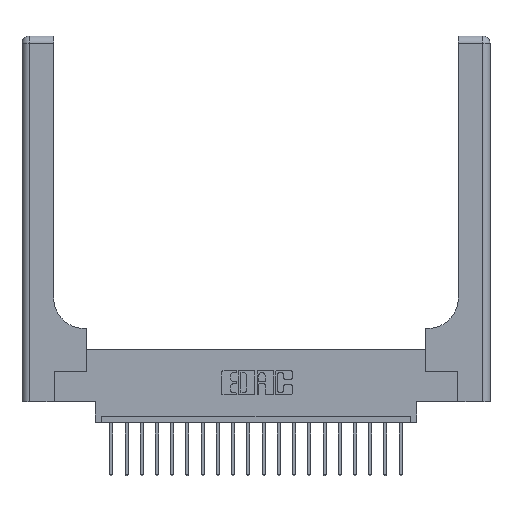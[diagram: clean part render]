
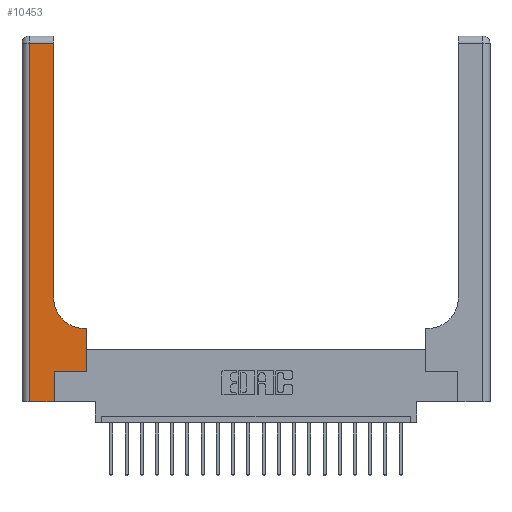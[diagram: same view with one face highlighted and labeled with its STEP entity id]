
A CAD part, top view. The second image highlights one B-rep face of the part: STEP entity #10453.
In plain terms, the highlighted planar face has unit normal (0, 0, 1).
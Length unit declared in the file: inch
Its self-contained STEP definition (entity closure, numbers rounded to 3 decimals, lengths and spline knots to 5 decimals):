
#412 = EDGE_CURVE ( 'NONE', #14794, #13893, #10977, .T. ) ;
#609 = DIRECTION ( 'NONE',  ( 1., 0., 0. ) ) ;
#1323 = VERTEX_POINT ( 'NONE', #8451 ) ;
#1460 = DIRECTION ( 'NONE',  ( 0., 0., -1. ) ) ;
#1505 = CARTESIAN_POINT ( 'NONE',  ( 0.06, 3., 0.37 ) ) ;
#1817 = ORIENTED_EDGE ( 'NONE', *, *, #3419, .T. ) ;
#2154 = ORIENTED_EDGE ( 'NONE', *, *, #20997, .T. ) ;
#2956 = CARTESIAN_POINT ( 'NONE',  ( 0., 3., 0.37 ) ) ;
#2967 = DIRECTION ( 'NONE',  ( 0., 1., 0. ) ) ;
#3419 = EDGE_CURVE ( 'NONE', #13768, #9009, #17662, .T. ) ;
#3520 = VECTOR ( 'NONE', #11251, 39.37008 ) ;
#3638 = VECTOR ( 'NONE', #9636, 39.37008 ) ;
#4428 = AXIS2_PLACEMENT_3D ( 'NONE', #9520, #8522, #15043 ) ;
#4526 = CARTESIAN_POINT ( 'NONE',  ( 0.06, 0., 0.37 ) ) ;
#4761 = VECTOR ( 'NONE', #16484, 39.37008 ) ;
#4892 = CARTESIAN_POINT ( 'NONE',  ( 0.528, 0.6, 0.37 ) ) ;
#5689 = VERTEX_POINT ( 'NONE', #10002 ) ;
#6119 = CARTESIAN_POINT ( 'NONE',  ( 0.26, 3., 0.37 ) ) ;
#6524 = VERTEX_POINT ( 'NONE', #8384 ) ;
#6579 = ORIENTED_EDGE ( 'NONE', *, *, #8821, .T. ) ;
#7042 = EDGE_CURVE ( 'NONE', #13893, #6524, #12755, .T. ) ;
#7211 = EDGE_LOOP ( 'NONE', ( #13120, #1817, #12132, #15295, #9755, #7879, #6579, #2154, #18688 ) ) ;
#7524 = EDGE_CURVE ( 'NONE', #5689, #1323, #10559, .T. ) ;
#7879 = ORIENTED_EDGE ( 'NONE', *, *, #7042, .T. ) ;
#7968 = DIRECTION ( 'NONE',  ( -1., 0., 0. ) ) ;
#8384 = CARTESIAN_POINT ( 'NONE',  ( 0.528, 0.25, 0.37 ) ) ;
#8451 = CARTESIAN_POINT ( 'NONE',  ( 0.26, 0.85, 0.37 ) ) ;
#8522 = DIRECTION ( 'NONE',  ( 0., 0., -1. ) ) ;
#8564 = LINE ( 'NONE', #18298, #4761 ) ;
#8821 = EDGE_CURVE ( 'NONE', #6524, #9029, #20652, .T. ) ;
#8977 = CARTESIAN_POINT ( 'NONE',  ( 0.528, 0.25, 0.37 ) ) ;
#9009 = VERTEX_POINT ( 'NONE', #19657 ) ;
#9029 = VERTEX_POINT ( 'NONE', #4892 ) ;
#9520 = CARTESIAN_POINT ( 'NONE',  ( 0.51, 0.85, 0.37 ) ) ;
#9636 = DIRECTION ( 'NONE',  ( -1., 0., 0. ) ) ;
#9755 = ORIENTED_EDGE ( 'NONE', *, *, #412, .T. ) ;
#10002 = CARTESIAN_POINT ( 'NONE',  ( 0.51, 0.6, 0.37 ) ) ;
#10453 = ADVANCED_FACE ( 'NONE', ( #11486 ), #17591, .F. ) ;
#10559 = CIRCLE ( 'NONE', #4428, 0.25 ) ;
#10977 = LINE ( 'NONE', #14181, #19838 ) ;
#11251 = DIRECTION ( 'NONE',  ( 1., 0., 0. ) ) ;
#11486 = FACE_OUTER_BOUND ( 'NONE', #7211, .T. ) ;
#12128 = VECTOR ( 'NONE', #12629, 39.37008 ) ;
#12132 = ORIENTED_EDGE ( 'NONE', *, *, #16173, .T. ) ;
#12240 = VECTOR ( 'NONE', #20337, 39.37008 ) ;
#12518 = EDGE_CURVE ( 'NONE', #1323, #13768, #17647, .T. ) ;
#12629 = DIRECTION ( 'NONE',  ( 0., 1., 0. ) ) ;
#12755 = LINE ( 'NONE', #19292, #3520 ) ;
#13120 = ORIENTED_EDGE ( 'NONE', *, *, #12518, .T. ) ;
#13768 = VERTEX_POINT ( 'NONE', #21093 ) ;
#13893 = VERTEX_POINT ( 'NONE', #19901 ) ;
#14181 = CARTESIAN_POINT ( 'NONE',  ( 0.265, 0., 0.37 ) ) ;
#14653 = VERTEX_POINT ( 'NONE', #4526 ) ;
#14794 = VERTEX_POINT ( 'NONE', #15188 ) ;
#14919 = CARTESIAN_POINT ( 'NONE',  ( 0., 0., 0.37 ) ) ;
#15043 = DIRECTION ( 'NONE',  ( 1., 0., 0. ) ) ;
#15188 = CARTESIAN_POINT ( 'NONE',  ( 0.265, 0., 0.37 ) ) ;
#15239 = LINE ( 'NONE', #14919, #17337 ) ;
#15295 = ORIENTED_EDGE ( 'NONE', *, *, #18822, .T. ) ;
#16173 = EDGE_CURVE ( 'NONE', #9009, #14653, #17850, .T. ) ;
#16469 = DIRECTION ( 'NONE',  ( 0., -1., 0. ) ) ;
#16484 = DIRECTION ( 'NONE',  ( -1., 0., 0. ) ) ;
#17337 = VECTOR ( 'NONE', #609, 39.37008 ) ;
#17591 = PLANE ( 'NONE',  #20380 ) ;
#17647 = LINE ( 'NONE', #6119, #12128 ) ;
#17662 = LINE ( 'NONE', #20902, #3638 ) ;
#17850 = LINE ( 'NONE', #1505, #18330 ) ;
#18298 = CARTESIAN_POINT ( 'NONE',  ( 0.26, 0.6, 0.37 ) ) ;
#18330 = VECTOR ( 'NONE', #16469, 39.37008 ) ;
#18688 = ORIENTED_EDGE ( 'NONE', *, *, #7524, .T. ) ;
#18822 = EDGE_CURVE ( 'NONE', #14653, #14794, #15239, .T. ) ;
#19292 = CARTESIAN_POINT ( 'NONE',  ( 0.265, 0.25, 0.37 ) ) ;
#19657 = CARTESIAN_POINT ( 'NONE',  ( 0.06, 2.94, 0.37 ) ) ;
#19838 = VECTOR ( 'NONE', #2967, 39.37008 ) ;
#19901 = CARTESIAN_POINT ( 'NONE',  ( 0.265, 0.25, 0.37 ) ) ;
#20337 = DIRECTION ( 'NONE',  ( 0., 1., 0. ) ) ;
#20380 = AXIS2_PLACEMENT_3D ( 'NONE', #2956, #1460, #7968 ) ;
#20652 = LINE ( 'NONE', #8977, #12240 ) ;
#20902 = CARTESIAN_POINT ( 'NONE',  ( 0., 2.94, 0.37 ) ) ;
#20997 = EDGE_CURVE ( 'NONE', #9029, #5689, #8564, .T. ) ;
#21093 = CARTESIAN_POINT ( 'NONE',  ( 0.26, 2.94, 0.37 ) ) ;
